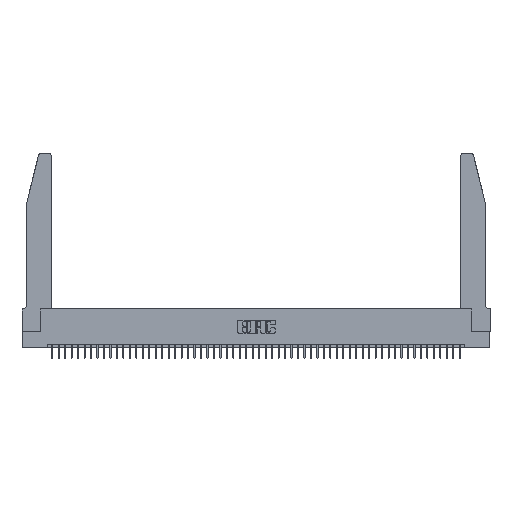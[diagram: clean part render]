
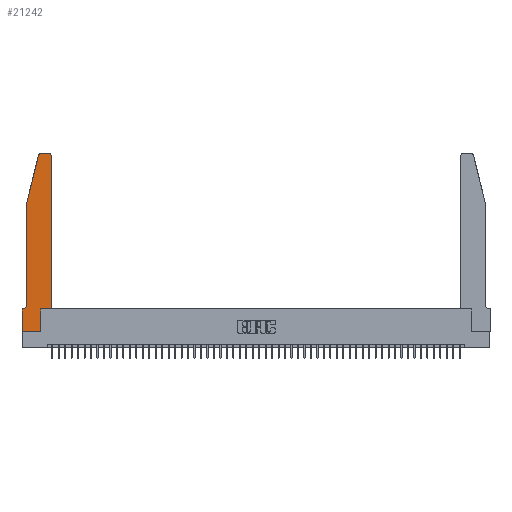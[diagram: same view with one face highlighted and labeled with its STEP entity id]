
A CAD part, top view. The second image highlights one B-rep face of the part: STEP entity #21242.
In plain terms, the highlighted planar face has unit normal (0, 0, 1).
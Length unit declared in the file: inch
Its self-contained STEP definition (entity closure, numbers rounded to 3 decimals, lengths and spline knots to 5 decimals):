
#211 = LINE ( 'NONE', #26273, #31191 ) ;
#736 = VERTEX_POINT ( 'NONE', #11696 ) ;
#775 = EDGE_CURVE ( 'NONE', #41452, #34478, #17362, .T. ) ;
#1115 = EDGE_CURVE ( 'NONE', #45495, #6604, #211, .T. ) ;
#1760 = ORIENTED_EDGE ( 'NONE', *, *, #5063, .T. ) ;
#3670 = ORIENTED_EDGE ( 'NONE', *, *, #50529, .T. ) ;
#3714 = CARTESIAN_POINT ( 'NONE',  ( 0.4505, 0.35, 0.37 ) ) ;
#3721 = VECTOR ( 'NONE', #47853, 39.37008 ) ;
#3882 = CARTESIAN_POINT ( 'NONE',  ( 0., 0.35, 0.37 ) ) ;
#4823 = AXIS2_PLACEMENT_3D ( 'NONE', #35796, #11692, #39777 ) ;
#5063 = EDGE_CURVE ( 'NONE', #736, #45495, #13899, .T. ) ;
#6147 = VECTOR ( 'NONE', #20917, 39.37008 ) ;
#6604 = VERTEX_POINT ( 'NONE', #27507 ) ;
#8712 = ORIENTED_EDGE ( 'NONE', *, *, #44143, .T. ) ;
#8758 = LINE ( 'NONE', #17919, #51423 ) ;
#9689 = CARTESIAN_POINT ( 'NONE',  ( 0.0755, 0.35, 0.37 ) ) ;
#10036 = CIRCLE ( 'NONE', #4823, 0.03 ) ;
#10405 = PLANE ( 'NONE',  #12437 ) ;
#11501 = DIRECTION ( 'NONE',  ( 0., 0., -1. ) ) ;
#11692 = DIRECTION ( 'NONE',  ( 0., 0., 1. ) ) ;
#11696 = CARTESIAN_POINT ( 'NONE',  ( 0.0055, 0.35, 0.37 ) ) ;
#11910 = ORIENTED_EDGE ( 'NONE', *, *, #33044, .T. ) ;
#12437 = AXIS2_PLACEMENT_3D ( 'NONE', #26280, #38519, #14509 ) ;
#12572 = EDGE_CURVE ( 'NONE', #38767, #736, #47101, .T. ) ;
#13125 = VECTOR ( 'NONE', #30962, 39.37008 ) ;
#13739 = EDGE_CURVE ( 'NONE', #6604, #34357, #15670, .T. ) ;
#13899 = LINE ( 'NONE', #9689, #25853 ) ;
#14344 = DIRECTION ( 'NONE',  ( 0., -1., 0. ) ) ;
#14509 = DIRECTION ( 'NONE',  ( 1., 0., 0. ) ) ;
#15475 = CARTESIAN_POINT ( 'NONE',  ( 0.2865, 0.35, 0.37 ) ) ;
#15670 = LINE ( 'NONE', #44864, #6147 ) ;
#16730 = VERTEX_POINT ( 'NONE', #35117 ) ;
#17362 = LINE ( 'NONE', #3714, #27464 ) ;
#17674 = VERTEX_POINT ( 'NONE', #28864 ) ;
#17919 = CARTESIAN_POINT ( 'NONE',  ( 0.0755, 2., 0.37 ) ) ;
#18258 = ORIENTED_EDGE ( 'NONE', *, *, #12572, .T. ) ;
#18315 = ORIENTED_EDGE ( 'NONE', *, *, #28381, .T. ) ;
#19264 = CARTESIAN_POINT ( 'NONE',  ( 0.4205, 2.75, 0.37 ) ) ;
#20757 = ORIENTED_EDGE ( 'NONE', *, *, #50955, .T. ) ;
#20917 = DIRECTION ( 'NONE',  ( 1., 0., 0. ) ) ;
#21242 = ADVANCED_FACE ( 'NONE', ( #39639 ), #10405, .T. ) ;
#21241 = DIRECTION ( 'NONE',  ( 0., 0., 1. ) ) ;
#21724 = CARTESIAN_POINT ( 'NONE',  ( 0.2865, 0.35, 0.37 ) ) ;
#21920 = LINE ( 'NONE', #15475, #32562 ) ;
#23344 = AXIS2_PLACEMENT_3D ( 'NONE', #35615, #11501, #39603 ) ;
#23987 = VECTOR ( 'NONE', #24288, 39.37008 ) ;
#24288 = DIRECTION ( 'NONE',  ( 1., 0., 0. ) ) ;
#25069 = VERTEX_POINT ( 'NONE', #21724 ) ;
#25853 = VECTOR ( 'NONE', #41848, 39.37008 ) ;
#26273 = CARTESIAN_POINT ( 'NONE',  ( 0., 0., 0.37 ) ) ;
#26280 = CARTESIAN_POINT ( 'NONE',  ( 0., 0.35, 0.37 ) ) ;
#26351 = LINE ( 'NONE', #39009, #13125 ) ;
#27464 = VECTOR ( 'NONE', #35965, 39.37008 ) ;
#27507 = CARTESIAN_POINT ( 'NONE',  ( 0., 0., 0.37 ) ) ;
#27721 = ORIENTED_EDGE ( 'NONE', *, *, #775, .T. ) ;
#28381 = EDGE_CURVE ( 'NONE', #34478, #51334, #10036, .T. ) ;
#28716 = CARTESIAN_POINT ( 'NONE',  ( 0.0755, 0.42, 0.37 ) ) ;
#28842 = CARTESIAN_POINT ( 'NONE',  ( 0.4505, 2.72, 0.37 ) ) ;
#28864 = CARTESIAN_POINT ( 'NONE',  ( 0.25487, 2.72718, 0.37 ) ) ;
#29462 = CARTESIAN_POINT ( 'NONE',  ( 0.284, 2.75, 0.37 ) ) ;
#30962 = DIRECTION ( 'NONE',  ( -1., 0., 0. ) ) ;
#31191 = VECTOR ( 'NONE', #14344, 39.37008 ) ;
#31428 = DIRECTION ( 'NONE',  ( 0., 1., 0. ) ) ;
#32562 = VECTOR ( 'NONE', #31428, 39.37008 ) ;
#33044 = EDGE_CURVE ( 'NONE', #17674, #16730, #46463, .T. ) ;
#33060 = EDGE_CURVE ( 'NONE', #25069, #41452, #34627, .T. ) ;
#34357 = VERTEX_POINT ( 'NONE', #44072 ) ;
#34478 = VERTEX_POINT ( 'NONE', #28842 ) ;
#34567 = EDGE_LOOP ( 'NONE', ( #8712, #20757, #11910, #3670, #18258, #1760, #44582, #45822, #49597, #45235, #27721, #18315 ) ) ;
#34627 = LINE ( 'NONE', #40193, #23987 ) ;
#35117 = CARTESIAN_POINT ( 'NONE',  ( 0.0755, 2., 0.37 ) ) ;
#35615 = CARTESIAN_POINT ( 'NONE',  ( 0.0055, 0.42, 0.37 ) ) ;
#35796 = CARTESIAN_POINT ( 'NONE',  ( 0.4205, 2.72, 0.37 ) ) ;
#35965 = DIRECTION ( 'NONE',  ( 0., 1., 0. ) ) ;
#36011 = CARTESIAN_POINT ( 'NONE',  ( 0.0755, 2., 0.37 ) ) ;
#37891 = DIRECTION ( 'NONE',  ( 0., -1., 0. ) ) ;
#38519 = DIRECTION ( 'NONE',  ( 0., 0., 1. ) ) ;
#38767 = VERTEX_POINT ( 'NONE', #28716 ) ;
#39009 = CARTESIAN_POINT ( 'NONE',  ( 0.2605, 2.75, 0.37 ) ) ;
#39603 = DIRECTION ( 'NONE',  ( -1., 0., 0. ) ) ;
#39639 = FACE_OUTER_BOUND ( 'NONE', #34567, .T. ) ;
#39777 = DIRECTION ( 'NONE',  ( 1., 0., 0. ) ) ;
#40193 = CARTESIAN_POINT ( 'NONE',  ( 0.4505, 0.35, 0.37 ) ) ;
#41452 = VERTEX_POINT ( 'NONE', #51805 ) ;
#41848 = DIRECTION ( 'NONE',  ( -1., 0., 0. ) ) ;
#44072 = CARTESIAN_POINT ( 'NONE',  ( 0.2865, 0., 0.37 ) ) ;
#44143 = EDGE_CURVE ( 'NONE', #51334, #45172, #26351, .T. ) ;
#44582 = ORIENTED_EDGE ( 'NONE', *, *, #1115, .T. ) ;
#44852 = EDGE_CURVE ( 'NONE', #34357, #25069, #21920, .T. ) ;
#44864 = CARTESIAN_POINT ( 'NONE',  ( 0., 0., 0.37 ) ) ;
#45053 = AXIS2_PLACEMENT_3D ( 'NONE', #45176, #21241, #49183 ) ;
#45172 = VERTEX_POINT ( 'NONE', #29462 ) ;
#45176 = CARTESIAN_POINT ( 'NONE',  ( 0.284, 2.72, 0.37 ) ) ;
#45235 = ORIENTED_EDGE ( 'NONE', *, *, #33060, .T. ) ;
#45495 = VERTEX_POINT ( 'NONE', #3882 ) ;
#45772 = CIRCLE ( 'NONE', #45053, 0.03 ) ;
#45822 = ORIENTED_EDGE ( 'NONE', *, *, #13739, .T. ) ;
#46463 = LINE ( 'NONE', #36011, #3721 ) ;
#47101 = CIRCLE ( 'NONE', #23344, 0.07 ) ;
#47853 = DIRECTION ( 'NONE',  ( -0.239, -0.971, 0. ) ) ;
#49183 = DIRECTION ( 'NONE',  ( 1., 0., 0. ) ) ;
#49597 = ORIENTED_EDGE ( 'NONE', *, *, #44852, .T. ) ;
#50529 = EDGE_CURVE ( 'NONE', #16730, #38767, #8758, .T. ) ;
#50955 = EDGE_CURVE ( 'NONE', #45172, #17674, #45772, .T. ) ;
#51334 = VERTEX_POINT ( 'NONE', #19264 ) ;
#51423 = VECTOR ( 'NONE', #37891, 39.37008 ) ;
#51805 = CARTESIAN_POINT ( 'NONE',  ( 0.4505, 0.35, 0.37 ) ) ;
